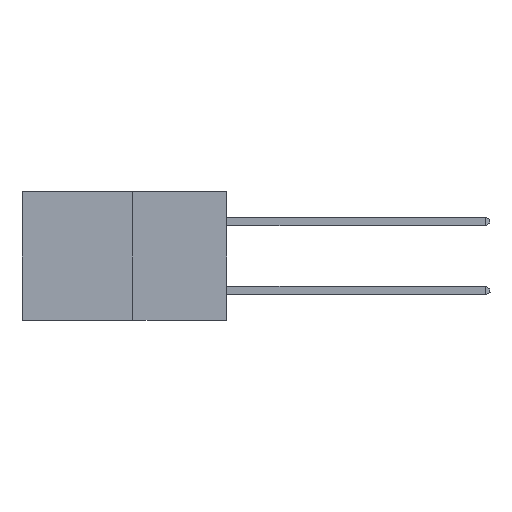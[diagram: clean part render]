
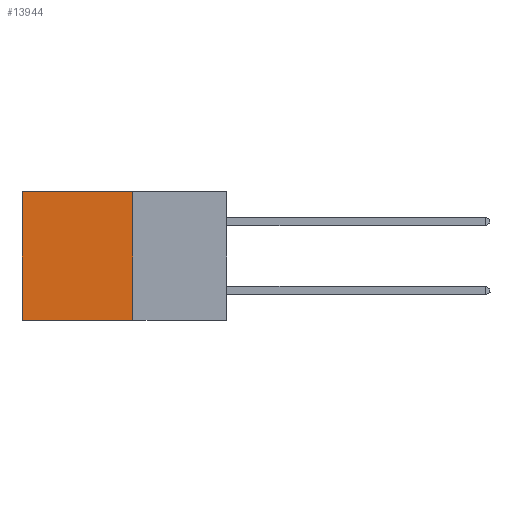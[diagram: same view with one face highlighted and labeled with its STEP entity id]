
A CAD part, left-side view. The second image highlights one B-rep face of the part: STEP entity #13944.
In plain terms, the highlighted planar face has unit normal (-1, 0, 0).
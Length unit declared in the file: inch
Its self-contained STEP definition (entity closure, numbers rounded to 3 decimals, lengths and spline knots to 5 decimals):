
#670 = DIRECTION ( 'NONE',  ( 0., 0., -1. ) ) ;
#2296 = VERTEX_POINT ( 'NONE', #22082 ) ;
#2801 = ORIENTED_EDGE ( 'NONE', *, *, #14587, .F. ) ;
#3439 = VECTOR ( 'NONE', #11130, 39.37008 ) ;
#3520 = EDGE_CURVE ( 'NONE', #12080, #20721, #5351, .T. ) ;
#4007 = LINE ( 'NONE', #9371, #3439 ) ;
#4257 = ORIENTED_EDGE ( 'NONE', *, *, #22585, .F. ) ;
#5351 = LINE ( 'NONE', #6915, #8986 ) ;
#6415 = CARTESIAN_POINT ( 'NONE',  ( 0.277, 0.59, -0.37 ) ) ;
#6567 = CARTESIAN_POINT ( 'NONE',  ( 0.277, 0.27, -0.37 ) ) ;
#6854 = DIRECTION ( 'NONE',  ( 0., 0., -1. ) ) ;
#6915 = CARTESIAN_POINT ( 'NONE',  ( 0.277, 0.59, -0.37 ) ) ;
#7932 = DIRECTION ( 'NONE',  ( 0., 1., 0. ) ) ;
#8166 = CARTESIAN_POINT ( 'NONE',  ( 0.277, 0.27, 0. ) ) ;
#8494 = ORIENTED_EDGE ( 'NONE', *, *, #14001, .T. ) ;
#8986 = VECTOR ( 'NONE', #6854, 39.37008 ) ;
#9371 = CARTESIAN_POINT ( 'NONE',  ( 0.277, 0.27, -0.37 ) ) ;
#10591 = ORIENTED_EDGE ( 'NONE', *, *, #3520, .T. ) ;
#11130 = DIRECTION ( 'NONE',  ( 0., 0., -1. ) ) ;
#11306 = DIRECTION ( 'NONE',  ( 1., 0., 0. ) ) ;
#11524 = FACE_OUTER_BOUND ( 'NONE', #20921, .T. ) ;
#12080 = VERTEX_POINT ( 'NONE', #18558 ) ;
#13944 = ADVANCED_FACE ( 'NONE', ( #11524 ), #16493, .F. ) ;
#14001 = EDGE_CURVE ( 'NONE', #14133, #12080, #19752, .T. ) ;
#14133 = VERTEX_POINT ( 'NONE', #8166 ) ;
#14173 = AXIS2_PLACEMENT_3D ( 'NONE', #21755, #11306, #670 ) ;
#14587 = EDGE_CURVE ( 'NONE', #14133, #2296, #4007, .T. ) ;
#15077 = VECTOR ( 'NONE', #7932, 39.37008 ) ;
#16493 = PLANE ( 'NONE',  #14173 ) ;
#16647 = CARTESIAN_POINT ( 'NONE',  ( 0.277, 0.27, 0. ) ) ;
#17697 = LINE ( 'NONE', #6567, #19622 ) ;
#18558 = CARTESIAN_POINT ( 'NONE',  ( 0.277, 0.59, 0. ) ) ;
#19622 = VECTOR ( 'NONE', #22321, 39.37008 ) ;
#19752 = LINE ( 'NONE', #16647, #15077 ) ;
#20721 = VERTEX_POINT ( 'NONE', #6415 ) ;
#20921 = EDGE_LOOP ( 'NONE', ( #10591, #4257, #2801, #8494 ) ) ;
#21755 = CARTESIAN_POINT ( 'NONE',  ( 0.277, 0.27, -0.37 ) ) ;
#22082 = CARTESIAN_POINT ( 'NONE',  ( 0.277, 0.27, -0.37 ) ) ;
#22321 = DIRECTION ( 'NONE',  ( 0., 1., 0. ) ) ;
#22585 = EDGE_CURVE ( 'NONE', #2296, #20721, #17697, .T. ) ;
